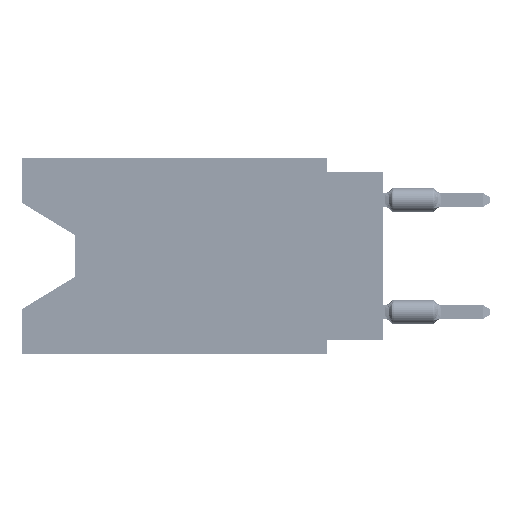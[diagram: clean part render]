
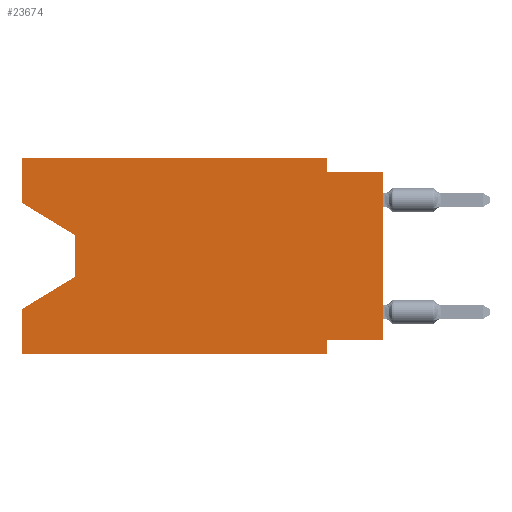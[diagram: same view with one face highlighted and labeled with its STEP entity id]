
A CAD part, left-side view. The second image highlights one B-rep face of the part: STEP entity #23674.
In plain terms, the highlighted planar face has unit normal (-1, 0, 0).
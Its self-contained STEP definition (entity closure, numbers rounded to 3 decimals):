
#157 = VECTOR ( 'NONE', #64826, 1000. ) ;
#398 = VERTEX_POINT ( 'NONE', #46171 ) ;
#552 = DIRECTION ( 'NONE',  ( 0., 1., 0. ) ) ;
#2087 = VERTEX_POINT ( 'NONE', #31182 ) ;
#2833 = VECTOR ( 'NONE', #552, 1000. ) ;
#3977 = CARTESIAN_POINT ( 'NONE',  ( 0., 16.383, -8.89 ) ) ;
#4650 = VERTEX_POINT ( 'NONE', #33229 ) ;
#5246 = CARTESIAN_POINT ( 'NONE',  ( 0., 16.383, -8.89 ) ) ;
#5344 = DIRECTION ( 'NONE',  ( 0., -0.855, -0.519 ) ) ;
#6051 = DIRECTION ( 'NONE',  ( 0., 0., -1. ) ) ;
#6153 = CARTESIAN_POINT ( 'NONE',  ( 0., 2.54, -8.89 ) ) ;
#6312 = DIRECTION ( 'NONE',  ( 0., 0.855, -0.519 ) ) ;
#7578 = CARTESIAN_POINT ( 'NONE',  ( 0., 16.383, 0. ) ) ;
#7643 = VERTEX_POINT ( 'NONE', #5246 ) ;
#7878 = PLANE ( 'NONE',  #13905 ) ;
#11384 = ORIENTED_EDGE ( 'NONE', *, *, #30582, .T. ) ;
#11678 = VECTOR ( 'NONE', #43633, 1000. ) ;
#13587 = VECTOR ( 'NONE', #16547, 1000. ) ;
#13905 = AXIS2_PLACEMENT_3D ( 'NONE', #57321, #19686, #19337 ) ;
#14208 = ORIENTED_EDGE ( 'NONE', *, *, #22242, .T. ) ;
#15813 = VECTOR ( 'NONE', #63299, 1000. ) ;
#16031 = ORIENTED_EDGE ( 'NONE', *, *, #25480, .F. ) ;
#16547 = DIRECTION ( 'NONE',  ( 0., 0., 1. ) ) ;
#16938 = CARTESIAN_POINT ( 'NONE',  ( 0., 2.54, 0. ) ) ;
#17127 = LINE ( 'NONE', #49725, #11678 ) ;
#17166 = CARTESIAN_POINT ( 'NONE',  ( 0., 2.54, -8.89 ) ) ;
#18279 = VERTEX_POINT ( 'NONE', #69341 ) ;
#18387 = VECTOR ( 'NONE', #61343, 1000. ) ;
#19337 = DIRECTION ( 'NONE',  ( 0., 0., -1. ) ) ;
#19686 = DIRECTION ( 'NONE',  ( 1., 0., 0. ) ) ;
#20827 = EDGE_CURVE ( 'NONE', #7643, #2087, #17127, .T. ) ;
#21962 = DIRECTION ( 'NONE',  ( 0., 0., -1. ) ) ;
#22242 = EDGE_CURVE ( 'NONE', #7643, #58626, #31569, .T. ) ;
#23674 = ADVANCED_FACE ( 'NONE', ( #35121 ), #7878, .F. ) ;
#24198 = CARTESIAN_POINT ( 'NONE',  ( 0., 0., -8.255 ) ) ;
#25328 = DIRECTION ( 'NONE',  ( 0., 0., -1. ) ) ;
#25480 = EDGE_CURVE ( 'NONE', #50740, #53212, #41824, .T. ) ;
#26652 = VERTEX_POINT ( 'NONE', #67853 ) ;
#27714 = EDGE_CURVE ( 'NONE', #30746, #4650, #31122, .T. ) ;
#29665 = EDGE_CURVE ( 'NONE', #26652, #398, #49193, .T. ) ;
#29944 = EDGE_CURVE ( 'NONE', #66094, #26652, #33293, .T. ) ;
#30582 = EDGE_CURVE ( 'NONE', #398, #2087, #50386, .T. ) ;
#30746 = VERTEX_POINT ( 'NONE', #24198 ) ;
#31122 = LINE ( 'NONE', #52984, #2833 ) ;
#31182 = CARTESIAN_POINT ( 'NONE',  ( 0., 16.383, -6.852 ) ) ;
#31217 = ORIENTED_EDGE ( 'NONE', *, *, #65289, .F. ) ;
#31569 = LINE ( 'NONE', #3977, #62152 ) ;
#32342 = CARTESIAN_POINT ( 'NONE',  ( 0., 13.97, -3.505 ) ) ;
#33030 = LINE ( 'NONE', #49160, #13587 ) ;
#33229 = CARTESIAN_POINT ( 'NONE',  ( 0., 2.54, -8.255 ) ) ;
#33293 = LINE ( 'NONE', #69840, #56949 ) ;
#34324 = CARTESIAN_POINT ( 'NONE',  ( 0., 16.383, -2.038 ) ) ;
#35121 = FACE_OUTER_BOUND ( 'NONE', #49755, .T. ) ;
#36594 = EDGE_CURVE ( 'NONE', #4650, #58626, #38674, .T. ) ;
#38674 = LINE ( 'NONE', #17166, #64068 ) ;
#38791 = ORIENTED_EDGE ( 'NONE', *, *, #40654, .F. ) ;
#39643 = CARTESIAN_POINT ( 'NONE',  ( 0., 13.97, -5.385 ) ) ;
#40199 = LINE ( 'NONE', #7578, #18387 ) ;
#40440 = ORIENTED_EDGE ( 'NONE', *, *, #42848, .T. ) ;
#40654 = EDGE_CURVE ( 'NONE', #66094, #18279, #57943, .T. ) ;
#41458 = CARTESIAN_POINT ( 'NONE',  ( 0., 16.383, 0. ) ) ;
#41824 = LINE ( 'NONE', #64721, #47201 ) ;
#42848 = EDGE_CURVE ( 'NONE', #30746, #54771, #33030, .T. ) ;
#43633 = DIRECTION ( 'NONE',  ( 0., 0., 1. ) ) ;
#45770 = ORIENTED_EDGE ( 'NONE', *, *, #29944, .T. ) ;
#45963 = ORIENTED_EDGE ( 'NONE', *, *, #48814, .F. ) ;
#46171 = CARTESIAN_POINT ( 'NONE',  ( 0., 13.97, -5.385 ) ) ;
#47001 = ORIENTED_EDGE ( 'NONE', *, *, #27714, .F. ) ;
#47201 = VECTOR ( 'NONE', #25328, 1000. ) ;
#48814 = EDGE_CURVE ( 'NONE', #18279, #50740, #40199, .T. ) ;
#49160 = CARTESIAN_POINT ( 'NONE',  ( 0., 0., 0. ) ) ;
#49193 = LINE ( 'NONE', #32342, #53481 ) ;
#49725 = CARTESIAN_POINT ( 'NONE',  ( 0., 16.383, 0. ) ) ;
#49755 = EDGE_LOOP ( 'NONE', ( #45770, #55033, #11384, #51624, #14208, #53303, #47001, #40440, #31217, #16031, #45963, #38791 ) ) ;
#50088 = VECTOR ( 'NONE', #6312, 1000. ) ;
#50386 = LINE ( 'NONE', #39643, #50088 ) ;
#50740 = VERTEX_POINT ( 'NONE', #16938 ) ;
#51624 = ORIENTED_EDGE ( 'NONE', *, *, #20827, .F. ) ;
#52984 = CARTESIAN_POINT ( 'NONE',  ( 0., 0., -8.255 ) ) ;
#53212 = VERTEX_POINT ( 'NONE', #65418 ) ;
#53303 = ORIENTED_EDGE ( 'NONE', *, *, #36594, .F. ) ;
#53481 = VECTOR ( 'NONE', #21962, 1000. ) ;
#53797 = DIRECTION ( 'NONE',  ( 0., -1., 0. ) ) ;
#54771 = VERTEX_POINT ( 'NONE', #62917 ) ;
#55033 = ORIENTED_EDGE ( 'NONE', *, *, #29665, .T. ) ;
#56949 = VECTOR ( 'NONE', #5344, 1000. ) ;
#57321 = CARTESIAN_POINT ( 'NONE',  ( 0., 16.383, 0. ) ) ;
#57943 = LINE ( 'NONE', #41458, #15813 ) ;
#58626 = VERTEX_POINT ( 'NONE', #6153 ) ;
#60522 = CARTESIAN_POINT ( 'NONE',  ( 0., 0., -0.635 ) ) ;
#61343 = DIRECTION ( 'NONE',  ( 0., -1., 0. ) ) ;
#62152 = VECTOR ( 'NONE', #53797, 1000. ) ;
#62917 = CARTESIAN_POINT ( 'NONE',  ( 0., 0., -0.635 ) ) ;
#63299 = DIRECTION ( 'NONE',  ( 0., 0., 1. ) ) ;
#64068 = VECTOR ( 'NONE', #6051, 1000. ) ;
#64721 = CARTESIAN_POINT ( 'NONE',  ( 0., 2.54, 0. ) ) ;
#64826 = DIRECTION ( 'NONE',  ( 0., -1., 0. ) ) ;
#65289 = EDGE_CURVE ( 'NONE', #53212, #54771, #69849, .T. ) ;
#65418 = CARTESIAN_POINT ( 'NONE',  ( 0., 2.54, -0.635 ) ) ;
#66094 = VERTEX_POINT ( 'NONE', #34324 ) ;
#67853 = CARTESIAN_POINT ( 'NONE',  ( 0., 13.97, -3.505 ) ) ;
#69341 = CARTESIAN_POINT ( 'NONE',  ( 0., 16.383, 0. ) ) ;
#69840 = CARTESIAN_POINT ( 'NONE',  ( 0., 16.383, -2.038 ) ) ;
#69849 = LINE ( 'NONE', #60522, #157 ) ;
